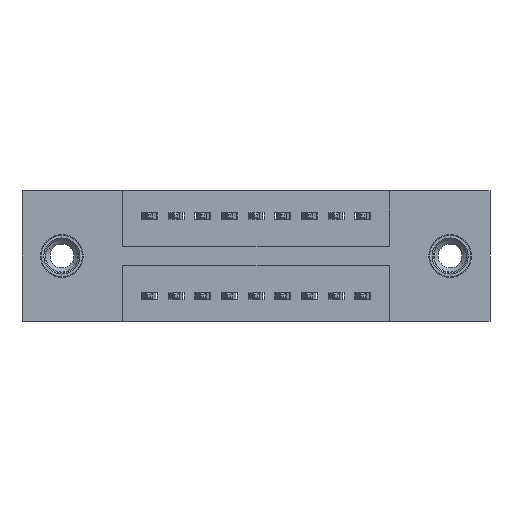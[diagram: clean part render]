
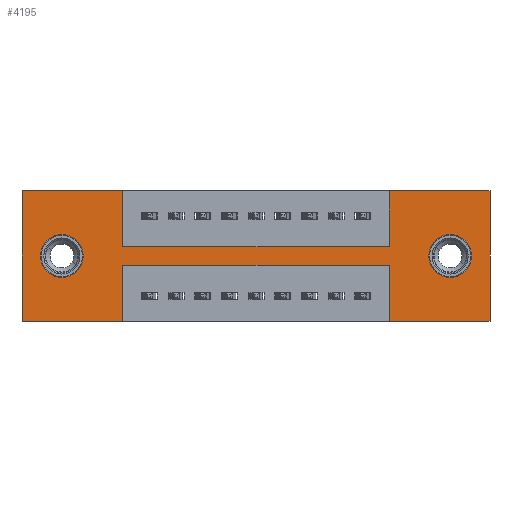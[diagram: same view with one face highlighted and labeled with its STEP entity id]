
A CAD part, front view. The second image highlights one B-rep face of the part: STEP entity #4195.
In plain terms, the highlighted planar face has unit normal (0, -1, 0).
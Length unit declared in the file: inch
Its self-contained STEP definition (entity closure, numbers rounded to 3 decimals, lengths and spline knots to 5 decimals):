
#14 = CARTESIAN_POINT ( 'NONE',  ( 0.1495, 0., -0.325 ) ) ;
#129 = VECTOR ( 'NONE', #7421, 39.37008 ) ;
#190 = CARTESIAN_POINT ( 'NONE',  ( 1.755, 0., -0.49 ) ) ;
#277 = LINE ( 'NONE', #6054, #11199 ) ;
#365 = VERTEX_POINT ( 'NONE', #2988 ) ;
#484 = DIRECTION ( 'NONE',  ( 0., 0., -1. ) ) ;
#530 = VECTOR ( 'NONE', #4774, 39.37008 ) ;
#645 = CARTESIAN_POINT ( 'NONE',  ( 1.6055, 0., -0.165 ) ) ;
#650 = CARTESIAN_POINT ( 'NONE',  ( 0., 0., -0.49 ) ) ;
#733 = CARTESIAN_POINT ( 'NONE',  ( 0., 0., 0. ) ) ;
#829 = AXIS2_PLACEMENT_3D ( 'NONE', #650, #2357, #5214 ) ;
#835 = LINE ( 'NONE', #7769, #6312 ) ;
#934 = ORIENTED_EDGE ( 'NONE', *, *, #10628, .F. ) ;
#973 = CARTESIAN_POINT ( 'NONE',  ( 1.3775, 0., -0.21 ) ) ;
#1057 = VECTOR ( 'NONE', #3038, 39.37008 ) ;
#1218 = CARTESIAN_POINT ( 'NONE',  ( 0., 0., -0.49 ) ) ;
#1282 = CARTESIAN_POINT ( 'NONE',  ( 1.3775, 0., -0.28 ) ) ;
#1348 = EDGE_CURVE ( 'NONE', #6797, #4147, #835, .T. ) ;
#1397 = CARTESIAN_POINT ( 'NONE',  ( 1.3775, 0., 0. ) ) ;
#1551 = CARTESIAN_POINT ( 'NONE',  ( 0.3775, 0., -0.28 ) ) ;
#1592 = DIRECTION ( 'NONE',  ( 0., 1., 0. ) ) ;
#1740 = DIRECTION ( 'NONE',  ( 0., 1., 0. ) ) ;
#1779 = CARTESIAN_POINT ( 'NONE',  ( 1.6055, 0., -0.245 ) ) ;
#2146 = ORIENTED_EDGE ( 'NONE', *, *, #9100, .T. ) ;
#2275 = VERTEX_POINT ( 'NONE', #4459 ) ;
#2357 = DIRECTION ( 'NONE',  ( 0., -1., 0. ) ) ;
#2372 = EDGE_CURVE ( 'NONE', #10475, #7002, #3539, .T. ) ;
#2486 = DIRECTION ( 'NONE',  ( 0., 0., -1. ) ) ;
#2573 = ORIENTED_EDGE ( 'NONE', *, *, #5297, .F. ) ;
#2625 = DIRECTION ( 'NONE',  ( 0., 1., 0. ) ) ;
#2868 = LINE ( 'NONE', #973, #129 ) ;
#2983 = VECTOR ( 'NONE', #484, 39.37008 ) ;
#2988 = CARTESIAN_POINT ( 'NONE',  ( 1.755, 0., 0. ) ) ;
#3038 = DIRECTION ( 'NONE',  ( 0., 0., 1. ) ) ;
#3081 = DIRECTION ( 'NONE',  ( -1., 0., 0. ) ) ;
#3111 = DIRECTION ( 'NONE',  ( 0., 0., -1. ) ) ;
#3155 = LINE ( 'NONE', #1551, #6704 ) ;
#3216 = DIRECTION ( 'NONE',  ( -1., 0., 0. ) ) ;
#3228 = EDGE_CURVE ( 'NONE', #6554, #9117, #7634, .T. ) ;
#3231 = ORIENTED_EDGE ( 'NONE', *, *, #9683, .F. ) ;
#3252 = ORIENTED_EDGE ( 'NONE', *, *, #7426, .F. ) ;
#3261 = CARTESIAN_POINT ( 'NONE',  ( 0.3775, 0., -0.49 ) ) ;
#3376 = LINE ( 'NONE', #1282, #1057 ) ;
#3539 = LINE ( 'NONE', #7897, #530 ) ;
#3565 = LINE ( 'NONE', #733, #10658 ) ;
#3751 = ORIENTED_EDGE ( 'NONE', *, *, #10103, .F. ) ;
#3790 = VERTEX_POINT ( 'NONE', #8140 ) ;
#3827 = LINE ( 'NONE', #10138, #6018 ) ;
#4145 = DIRECTION ( 'NONE',  ( 0., 0., -1. ) ) ;
#4147 = VERTEX_POINT ( 'NONE', #9357 ) ;
#4163 = CARTESIAN_POINT ( 'NONE',  ( 1.6055, 0., -0.325 ) ) ;
#4195 = ADVANCED_FACE ( 'NONE', ( #10253, #10940, #4965 ), #10157, .T. ) ;
#4208 = CARTESIAN_POINT ( 'NONE',  ( 0.1495, 0., -0.245 ) ) ;
#4264 = VERTEX_POINT ( 'NONE', #4357 ) ;
#4287 = CARTESIAN_POINT ( 'NONE',  ( 0., 0., 0. ) ) ;
#4357 = CARTESIAN_POINT ( 'NONE',  ( 0., 0., -0.49 ) ) ;
#4381 = AXIS2_PLACEMENT_3D ( 'NONE', #9183, #5605, #3111 ) ;
#4441 = EDGE_CURVE ( 'NONE', #4147, #3790, #5361, .T. ) ;
#4459 = CARTESIAN_POINT ( 'NONE',  ( 1.3775, 0., -0.28 ) ) ;
#4464 = AXIS2_PLACEMENT_3D ( 'NONE', #10365, #2625, #11258 ) ;
#4774 = DIRECTION ( 'NONE',  ( -1., 0., 0. ) ) ;
#4965 = FACE_OUTER_BOUND ( 'NONE', #9470, .T. ) ;
#5019 = VERTEX_POINT ( 'NONE', #645 ) ;
#5214 = DIRECTION ( 'NONE',  ( 0., 0., -1. ) ) ;
#5297 = EDGE_CURVE ( 'NONE', #9117, #4264, #10372, .T. ) ;
#5351 = VECTOR ( 'NONE', #3081, 39.37008 ) ;
#5361 = LINE ( 'NONE', #6841, #7137 ) ;
#5605 = DIRECTION ( 'NONE',  ( 0., 1., 0. ) ) ;
#5731 = CARTESIAN_POINT ( 'NONE',  ( 0.3775, 0., -0.28 ) ) ;
#5759 = ORIENTED_EDGE ( 'NONE', *, *, #9702, .T. ) ;
#5934 = CARTESIAN_POINT ( 'NONE',  ( 0.1495, 0., -0.165 ) ) ;
#5942 = ORIENTED_EDGE ( 'NONE', *, *, #2372, .F. ) ;
#6018 = VECTOR ( 'NONE', #8412, 39.37008 ) ;
#6054 = CARTESIAN_POINT ( 'NONE',  ( 0., 0., 0. ) ) ;
#6058 = CARTESIAN_POINT ( 'NONE',  ( 1.3775, 0., -0.49 ) ) ;
#6095 = CARTESIAN_POINT ( 'NONE',  ( 1.755, 0., 0. ) ) ;
#6113 = EDGE_LOOP ( 'NONE', ( #7766, #5759 ) ) ;
#6296 = AXIS2_PLACEMENT_3D ( 'NONE', #1779, #1740, #4145 ) ;
#6312 = VECTOR ( 'NONE', #10347, 39.37008 ) ;
#6493 = VECTOR ( 'NONE', #2486, 39.37008 ) ;
#6554 = VERTEX_POINT ( 'NONE', #10105 ) ;
#6601 = VERTEX_POINT ( 'NONE', #4163 ) ;
#6604 = ORIENTED_EDGE ( 'NONE', *, *, #9210, .F. ) ;
#6704 = VECTOR ( 'NONE', #3216, 39.37008 ) ;
#6765 = DIRECTION ( 'NONE',  ( 0., 0., 1. ) ) ;
#6797 = VERTEX_POINT ( 'NONE', #6872 ) ;
#6841 = CARTESIAN_POINT ( 'NONE',  ( 0.3775, 0., -0.21 ) ) ;
#6872 = CARTESIAN_POINT ( 'NONE',  ( 0.3775, 0., 0. ) ) ;
#6919 = DIRECTION ( 'NONE',  ( 1., 0., 0. ) ) ;
#6951 = DIRECTION ( 'NONE',  ( 1., 0., 0. ) ) ;
#7002 = VERTEX_POINT ( 'NONE', #6058 ) ;
#7137 = VECTOR ( 'NONE', #6951, 39.37008 ) ;
#7421 = DIRECTION ( 'NONE',  ( 0., 0., 1. ) ) ;
#7426 = EDGE_CURVE ( 'NONE', #365, #10475, #9088, .T. ) ;
#7529 = CIRCLE ( 'NONE', #4464, 0.08 ) ;
#7634 = LINE ( 'NONE', #5731, #2983 ) ;
#7766 = ORIENTED_EDGE ( 'NONE', *, *, #7968, .T. ) ;
#7769 = CARTESIAN_POINT ( 'NONE',  ( 0.3775, 0., -0.21 ) ) ;
#7897 = CARTESIAN_POINT ( 'NONE',  ( 0., 0., -0.49 ) ) ;
#7968 = EDGE_CURVE ( 'NONE', #11111, #10859, #9072, .T. ) ;
#8140 = CARTESIAN_POINT ( 'NONE',  ( 1.3775, 0., -0.21 ) ) ;
#8412 = DIRECTION ( 'NONE',  ( 1., 0., 0. ) ) ;
#8490 = CIRCLE ( 'NONE', #4381, 0.08 ) ;
#8552 = DIRECTION ( 'NONE',  ( 0., 0., 1. ) ) ;
#8725 = ORIENTED_EDGE ( 'NONE', *, *, #4441, .F. ) ;
#8941 = EDGE_CURVE ( 'NONE', #5019, #6601, #11071, .T. ) ;
#8970 = ORIENTED_EDGE ( 'NONE', *, *, #1348, .F. ) ;
#9072 = CIRCLE ( 'NONE', #10285, 0.08 ) ;
#9088 = LINE ( 'NONE', #6095, #6493 ) ;
#9100 = EDGE_CURVE ( 'NONE', #6601, #5019, #8490, .T. ) ;
#9117 = VERTEX_POINT ( 'NONE', #3261 ) ;
#9183 = CARTESIAN_POINT ( 'NONE',  ( 1.6055, 0., -0.245 ) ) ;
#9210 = EDGE_CURVE ( 'NONE', #4264, #11177, #3565, .T. ) ;
#9357 = CARTESIAN_POINT ( 'NONE',  ( 0.3775, 0., -0.21 ) ) ;
#9470 = EDGE_LOOP ( 'NONE', ( #3751, #8725, #8970, #9765, #6604, #2573, #10900, #3231, #934, #5942, #3252, #11018 ) ) ;
#9683 = EDGE_CURVE ( 'NONE', #2275, #6554, #3155, .T. ) ;
#9702 = EDGE_CURVE ( 'NONE', #10859, #11111, #7529, .T. ) ;
#9765 = ORIENTED_EDGE ( 'NONE', *, *, #10320, .F. ) ;
#9896 = EDGE_LOOP ( 'NONE', ( #10756, #2146 ) ) ;
#9913 = EDGE_CURVE ( 'NONE', #9915, #365, #3827, .T. ) ;
#9915 = VERTEX_POINT ( 'NONE', #1397 ) ;
#10103 = EDGE_CURVE ( 'NONE', #3790, #9915, #2868, .T. ) ;
#10105 = CARTESIAN_POINT ( 'NONE',  ( 0.3775, 0., -0.28 ) ) ;
#10138 = CARTESIAN_POINT ( 'NONE',  ( 0., 0., 0. ) ) ;
#10157 = PLANE ( 'NONE',  #829 ) ;
#10253 = FACE_BOUND ( 'NONE', #9896, .T. ) ;
#10285 = AXIS2_PLACEMENT_3D ( 'NONE', #4208, #1592, #6765 ) ;
#10320 = EDGE_CURVE ( 'NONE', #11177, #6797, #277, .T. ) ;
#10347 = DIRECTION ( 'NONE',  ( 0., 0., -1. ) ) ;
#10365 = CARTESIAN_POINT ( 'NONE',  ( 0.1495, 0., -0.245 ) ) ;
#10372 = LINE ( 'NONE', #1218, #5351 ) ;
#10475 = VERTEX_POINT ( 'NONE', #190 ) ;
#10628 = EDGE_CURVE ( 'NONE', #7002, #2275, #3376, .T. ) ;
#10658 = VECTOR ( 'NONE', #8552, 39.37008 ) ;
#10756 = ORIENTED_EDGE ( 'NONE', *, *, #8941, .T. ) ;
#10859 = VERTEX_POINT ( 'NONE', #14 ) ;
#10900 = ORIENTED_EDGE ( 'NONE', *, *, #3228, .F. ) ;
#10940 = FACE_BOUND ( 'NONE', #6113, .T. ) ;
#11018 = ORIENTED_EDGE ( 'NONE', *, *, #9913, .F. ) ;
#11071 = CIRCLE ( 'NONE', #6296, 0.08 ) ;
#11111 = VERTEX_POINT ( 'NONE', #5934 ) ;
#11177 = VERTEX_POINT ( 'NONE', #4287 ) ;
#11199 = VECTOR ( 'NONE', #6919, 39.37008 ) ;
#11258 = DIRECTION ( 'NONE',  ( 0., 0., 1. ) ) ;
